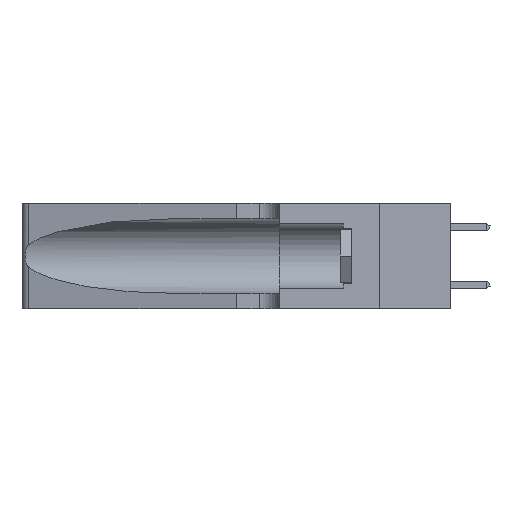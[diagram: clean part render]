
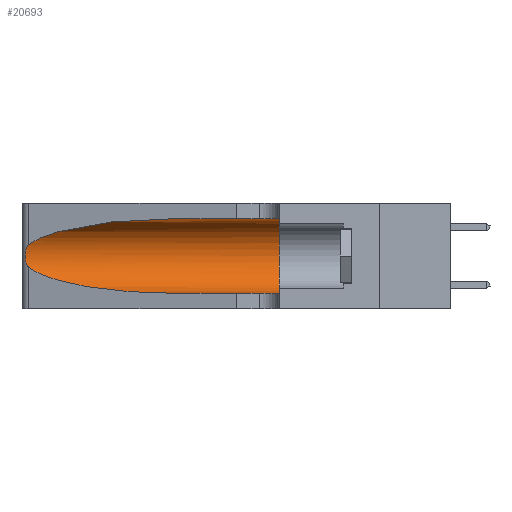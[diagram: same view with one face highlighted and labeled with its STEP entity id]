
A CAD part, left-side view. The second image highlights one B-rep face of the part: STEP entity #20693.
In plain terms, the highlighted cylindrical face has radius 3.308 mm (diameter 6.617 mm), a partial arc.
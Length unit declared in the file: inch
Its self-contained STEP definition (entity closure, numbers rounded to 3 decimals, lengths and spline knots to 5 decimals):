
#417 = CARTESIAN_POINT ( 'NONE',  ( 0.25487, 1.22718, 0.22369 ) ) ;
#741 = VERTEX_POINT ( 'NONE', #20259 ) ;
#1272 = CARTESIAN_POINT ( 'NONE',  ( 0.18966, 0.96281, 0.05475 ) ) ;
#1286 = DIRECTION ( 'NONE',  ( 0., -1., 0. ) ) ;
#1969 = CARTESIAN_POINT ( 'NONE',  ( 0.25789, 1.23486, 0.15765 ) ) ;
#2387 = CARTESIAN_POINT ( 'NONE',  ( 0.25639, 1.23186, 0.15144 ) ) ;
#2762 = CARTESIAN_POINT ( 'NONE',  ( 0.1305, 0.72297, 0.31525 ) ) ;
#2827 = AXIS2_PLACEMENT_3D ( 'NONE', #12962, #12682, #3323 ) ;
#3323 = DIRECTION ( 'NONE',  ( 0., 0., 1. ) ) ;
#4209 = CARTESIAN_POINT ( 'NONE',  ( 0.25555, 1.22994, 0.2215 ) ) ;
#5000 = CARTESIAN_POINT ( 'NONE',  ( 0.2373, 1.15595, 0.28018 ) ) ;
#5351 = LINE ( 'NONE', #7234, #14899 ) ;
#6172 = CARTESIAN_POINT ( 'NONE',  ( 0.1305, 1.61858, 0.31525 ) ) ;
#6178 = CARTESIAN_POINT ( 'NONE',  ( 0.26017, 1.23833, 0.17102 ) ) ;
#6366 = CARTESIAN_POINT ( 'NONE',  ( 0.26075, 1.23896, 0.178 ) ) ;
#7234 = CARTESIAN_POINT ( 'NONE',  ( 0.1305, 1.61858, 0.05475 ) ) ;
#7239 = CARTESIAN_POINT ( 'NONE',  ( 0.1305, 0.35, 0.31525 ) ) ;
#7498 = CARTESIAN_POINT ( 'NONE',  ( 0.1305, 1.61858, 0.185 ) ) ;
#8512 = VERTEX_POINT ( 'NONE', #13830 ) ;
#9265 = CARTESIAN_POINT ( 'NONE',  ( 0.25639, 1.23184, 0.21858 ) ) ;
#11034 = VERTEX_POINT ( 'NONE', #17902 ) ;
#11039 = EDGE_LOOP ( 'NONE', ( #20361, #23107, #17651, #20616, #22880, #23496 ) ) ;
#11676 = CARTESIAN_POINT ( 'NONE',  ( 0.18966, 0.96281, 0.31525 ) ) ;
#11813 = CIRCLE ( 'NONE', #2827, 0.13025 ) ;
#12682 = DIRECTION ( 'NONE',  ( 0., 1., 0. ) ) ;
#12712 = EDGE_CURVE ( 'NONE', #19434, #11034, #20346, .T. ) ;
#12962 = CARTESIAN_POINT ( 'NONE',  ( 0.1305, 0.35, 0.185 ) ) ;
#13830 = CARTESIAN_POINT ( 'NONE',  ( 0.25487, 1.22718, 0.22369 ) ) ;
#13878 = DIRECTION ( 'NONE',  ( 0., -1., 0. ) ) ;
#14208 = FACE_OUTER_BOUND ( 'NONE', #11039, .T. ) ;
#14246 = CARTESIAN_POINT ( 'NONE',  ( 0.2373, 1.15595, 0.08982 ) ) ;
#14625 = EDGE_CURVE ( 'NONE', #8512, #19434, #24639, .T. ) ;
#14769 = CARTESIAN_POINT ( 'NONE',  ( 0.25555, 1.22993, 0.14849 ) ) ;
#14899 = VECTOR ( 'NONE', #13878, 39.37008 ) ;
#16442 = CARTESIAN_POINT ( 'NONE',  ( 0.1305, 0.72297, 0.05475 ) ) ;
#16699 =( BOUNDED_CURVE ( )  B_SPLINE_CURVE ( 3, ( #2762, #11676, #5000, #17860 ),
 .UNSPECIFIED., .F., .T. ) 
 B_SPLINE_CURVE_WITH_KNOTS ( ( 4, 4 ),
 ( 1.5708, 2.84003 ),
 .UNSPECIFIED. ) 
 CURVE ( )  GEOMETRIC_REPRESENTATION_ITEM ( )  RATIONAL_B_SPLINE_CURVE ( ( 1., 0.87, 0.87, 1. ) ) 
 REPRESENTATION_ITEM ( '' )  );
#16719 = CARTESIAN_POINT ( 'NONE',  ( 0.25487, 1.22718, 0.14631 ) ) ;
#16960 = CARTESIAN_POINT ( 'NONE',  ( 0.25487, 1.22718, 0.14631 ) ) ;
#17209 = CARTESIAN_POINT ( 'NONE',  ( 0.25487, 1.22718, 0.14631 ) ) ;
#17492 = CARTESIAN_POINT ( 'NONE',  ( 0.25787, 1.23484, 0.2124 ) ) ;
#17585 = CARTESIAN_POINT ( 'NONE',  ( 0.25854, 1.2359, 0.20912 ) ) ;
#17651 = ORIENTED_EDGE ( 'NONE', *, *, #12712, .T. ) ;
#17860 = CARTESIAN_POINT ( 'NONE',  ( 0.25487, 1.22718, 0.22369 ) ) ;
#17902 = CARTESIAN_POINT ( 'NONE',  ( 0.1305, 0.72297, 0.05475 ) ) ;
#17993 = CARTESIAN_POINT ( 'NONE',  ( 0.26018, 1.23835, 0.19895 ) ) ;
#18094 = EDGE_CURVE ( 'NONE', #741, #24176, #25827, .T. ) ;
#18765 = VECTOR ( 'NONE', #23748, 39.37008 ) ;
#19434 = VERTEX_POINT ( 'NONE', #17209 ) ;
#20259 = CARTESIAN_POINT ( 'NONE',  ( 0.1305, 0.72297, 0.31525 ) ) ;
#20346 =( BOUNDED_CURVE ( )  B_SPLINE_CURVE ( 3, ( #16719, #14246, #1272, #16442 ),
 .UNSPECIFIED., .F., .F. ) 
 B_SPLINE_CURVE_WITH_KNOTS ( ( 4, 4 ),
 ( 3.44316, 4.71239 ),
 .UNSPECIFIED. ) 
 CURVE ( )  GEOMETRIC_REPRESENTATION_ITEM ( )  RATIONAL_B_SPLINE_CURVE ( ( 1., 0.87, 0.87, 1. ) ) 
 REPRESENTATION_ITEM ( '' )  );
#20361 = ORIENTED_EDGE ( 'NONE', *, *, #25640, .T. ) ;
#20616 = ORIENTED_EDGE ( 'NONE', *, *, #20670, .T. ) ;
#20670 = EDGE_CURVE ( 'NONE', #11034, #27436, #5351, .T. ) ;
#20693 = ADVANCED_FACE ( 'NONE', ( #14208 ), #26346, .F. ) ;
#20934 = EDGE_CURVE ( 'NONE', #24176, #27436, #11813, .T. ) ;
#22832 = AXIS2_PLACEMENT_3D ( 'NONE', #7498, #1286, #24850 ) ;
#22880 = ORIENTED_EDGE ( 'NONE', *, *, #20934, .F. ) ;
#23107 = ORIENTED_EDGE ( 'NONE', *, *, #14625, .T. ) ;
#23496 = ORIENTED_EDGE ( 'NONE', *, *, #18094, .F. ) ;
#23582 = CARTESIAN_POINT ( 'NONE',  ( 0.25856, 1.23593, 0.16098 ) ) ;
#23727 = CARTESIAN_POINT ( 'NONE',  ( 0.1305, 0.35, 0.05475 ) ) ;
#23748 = DIRECTION ( 'NONE',  ( 0., -1., 0. ) ) ;
#24176 = VERTEX_POINT ( 'NONE', #7239 ) ;
#24639 = B_SPLINE_CURVE_WITH_KNOTS ( 'NONE', 3,
 ( #417, #4209, #9265, #17492, #17585, #17993, #27968, #6366, #6178, #23582, #1969, #2387, #14769, #16960 ),
 .UNSPECIFIED., .F., .F.,
 ( 4, 2, 2, 2, 2, 2, 4 ),
 ( 0., 0.00027, 0.00053, 0.00107, 0.0016, 0.00187, 0.00214 ),
 .UNSPECIFIED. ) ;
#24850 = DIRECTION ( 'NONE',  ( 0., 0., -1. ) ) ;
#25640 = EDGE_CURVE ( 'NONE', #741, #8512, #16699, .T. ) ;
#25827 = LINE ( 'NONE', #6172, #18765 ) ;
#26346 = CYLINDRICAL_SURFACE ( 'NONE', #22832, 0.13025 ) ;
#27436 = VERTEX_POINT ( 'NONE', #23727 ) ;
#27968 = CARTESIAN_POINT ( 'NONE',  ( 0.26075, 1.23896, 0.19203 ) ) ;
